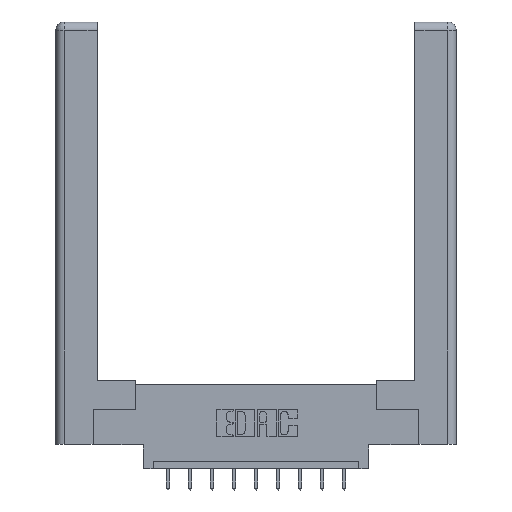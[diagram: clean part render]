
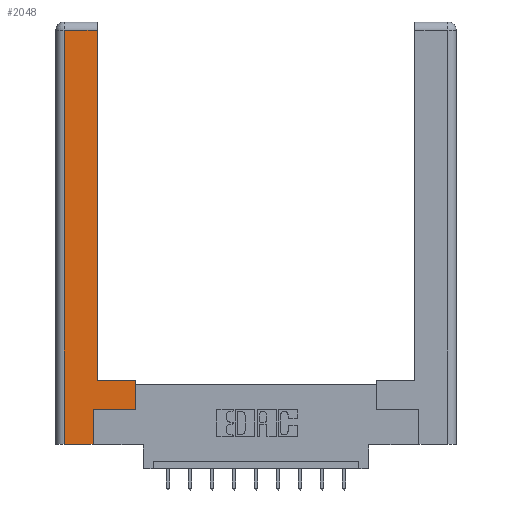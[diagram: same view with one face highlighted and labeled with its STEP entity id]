
A CAD part, top view. The second image highlights one B-rep face of the part: STEP entity #2048.
In plain terms, the highlighted planar face has unit normal (0, 0, 1).
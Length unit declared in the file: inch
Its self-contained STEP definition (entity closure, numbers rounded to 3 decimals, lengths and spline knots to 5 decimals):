
#720 = VERTEX_POINT ( 'NONE', #2684 ) ;
#749 = ORIENTED_EDGE ( 'NONE', *, *, #10631, .T. ) ;
#902 = FACE_OUTER_BOUND ( 'NONE', #11805, .T. ) ;
#1096 = VERTEX_POINT ( 'NONE', #10832 ) ;
#1123 = CARTESIAN_POINT ( 'NONE',  ( 0.295, 3., 0. ) ) ;
#1137 = VECTOR ( 'NONE', #4519, 39.37008 ) ;
#1896 = EDGE_CURVE ( 'NONE', #1096, #5167, #7364, .T. ) ;
#2048 = ADVANCED_FACE ( 'NONE', ( #902 ), #13759, .F. ) ;
#2146 = LINE ( 'NONE', #12828, #7787 ) ;
#2512 = EDGE_CURVE ( 'NONE', #6060, #3007, #8015, .T. ) ;
#2684 = CARTESIAN_POINT ( 'NONE',  ( 0.565, 0.245, 0. ) ) ;
#2881 = VECTOR ( 'NONE', #9727, 39.37008 ) ;
#2924 = VERTEX_POINT ( 'NONE', #7189 ) ;
#3007 = VERTEX_POINT ( 'NONE', #7711 ) ;
#4050 = DIRECTION ( 'NONE',  ( -1., 0., 0. ) ) ;
#4461 = VECTOR ( 'NONE', #7376, 39.37008 ) ;
#4519 = DIRECTION ( 'NONE',  ( -1., 0., 0. ) ) ;
#4553 = VECTOR ( 'NONE', #6603, 39.37008 ) ;
#4600 = EDGE_CURVE ( 'NONE', #7244, #720, #2146, .T. ) ;
#4672 = ORIENTED_EDGE ( 'NONE', *, *, #5648, .T. ) ;
#4952 = DIRECTION ( 'NONE',  ( 0., 1., 0. ) ) ;
#5167 = VERTEX_POINT ( 'NONE', #8017 ) ;
#5385 = EDGE_CURVE ( 'NONE', #2924, #6060, #6790, .T. ) ;
#5475 = DIRECTION ( 'NONE',  ( 0., 0., -1. ) ) ;
#5481 = DIRECTION ( 'NONE',  ( 0., 1., 0. ) ) ;
#5580 = CARTESIAN_POINT ( 'NONE',  ( 0.565, 0.45, 0. ) ) ;
#5648 = EDGE_CURVE ( 'NONE', #720, #2924, #6612, .T. ) ;
#5948 = ORIENTED_EDGE ( 'NONE', *, *, #7902, .T. ) ;
#6060 = VERTEX_POINT ( 'NONE', #8379 ) ;
#6286 = VECTOR ( 'NONE', #5481, 39.37008 ) ;
#6386 = LINE ( 'NONE', #9258, #11235 ) ;
#6537 = CARTESIAN_POINT ( 'NONE',  ( 0., 0., 0. ) ) ;
#6541 = ORIENTED_EDGE ( 'NONE', *, *, #4600, .T. ) ;
#6603 = DIRECTION ( 'NONE',  ( 1., 0., 0. ) ) ;
#6612 = LINE ( 'NONE', #5580, #6286 ) ;
#6633 = DIRECTION ( 'NONE',  ( -1., 0., 0. ) ) ;
#6790 = LINE ( 'NONE', #12006, #1137 ) ;
#7013 = VECTOR ( 'NONE', #4952, 39.37008 ) ;
#7189 = CARTESIAN_POINT ( 'NONE',  ( 0.565, 0.45, 0. ) ) ;
#7244 = VERTEX_POINT ( 'NONE', #12303 ) ;
#7364 = LINE ( 'NONE', #12982, #4553 ) ;
#7376 = DIRECTION ( 'NONE',  ( 0., -1., 0. ) ) ;
#7711 = CARTESIAN_POINT ( 'NONE',  ( 0.295, 2.94, 0. ) ) ;
#7787 = VECTOR ( 'NONE', #7946, 39.37008 ) ;
#7902 = EDGE_CURVE ( 'NONE', #3007, #8056, #6386, .T. ) ;
#7946 = DIRECTION ( 'NONE',  ( 1., 0., 0. ) ) ;
#8015 = LINE ( 'NONE', #1123, #2881 ) ;
#8017 = CARTESIAN_POINT ( 'NONE',  ( 0.265, 0., 0. ) ) ;
#8056 = VERTEX_POINT ( 'NONE', #10836 ) ;
#8379 = CARTESIAN_POINT ( 'NONE',  ( 0.295, 0.45, 0. ) ) ;
#8799 = LINE ( 'NONE', #11330, #7013 ) ;
#9081 = ORIENTED_EDGE ( 'NONE', *, *, #9083, .T. ) ;
#9083 = EDGE_CURVE ( 'NONE', #5167, #7244, #8799, .T. ) ;
#9258 = CARTESIAN_POINT ( 'NONE',  ( 0.0615, 2.94, 0. ) ) ;
#9727 = DIRECTION ( 'NONE',  ( 0., 1., 0. ) ) ;
#9917 = AXIS2_PLACEMENT_3D ( 'NONE', #6537, #5475, #6633 ) ;
#10112 = LINE ( 'NONE', #10612, #4461 ) ;
#10612 = CARTESIAN_POINT ( 'NONE',  ( 0.0615, 0., 0. ) ) ;
#10631 = EDGE_CURVE ( 'NONE', #8056, #1096, #10112, .T. ) ;
#10832 = CARTESIAN_POINT ( 'NONE',  ( 0.0615, 0., 0. ) ) ;
#10836 = CARTESIAN_POINT ( 'NONE',  ( 0.0615, 2.94, 0. ) ) ;
#11235 = VECTOR ( 'NONE', #4050, 39.37008 ) ;
#11330 = CARTESIAN_POINT ( 'NONE',  ( 0.265, 0.245, 0. ) ) ;
#11805 = EDGE_LOOP ( 'NONE', ( #13598, #5948, #749, #12336, #9081, #6541, #4672, #13114 ) ) ;
#12006 = CARTESIAN_POINT ( 'NONE',  ( 0.295, 0.45, 0. ) ) ;
#12303 = CARTESIAN_POINT ( 'NONE',  ( 0.265, 0.245, 0. ) ) ;
#12336 = ORIENTED_EDGE ( 'NONE', *, *, #1896, .T. ) ;
#12828 = CARTESIAN_POINT ( 'NONE',  ( 0.565, 0.245, 0. ) ) ;
#12982 = CARTESIAN_POINT ( 'NONE',  ( 0.265, 0., 0. ) ) ;
#13114 = ORIENTED_EDGE ( 'NONE', *, *, #5385, .T. ) ;
#13598 = ORIENTED_EDGE ( 'NONE', *, *, #2512, .T. ) ;
#13759 = PLANE ( 'NONE',  #9917 ) ;
